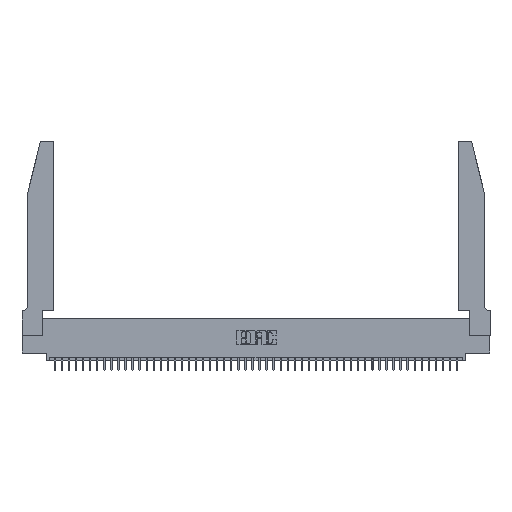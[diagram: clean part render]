
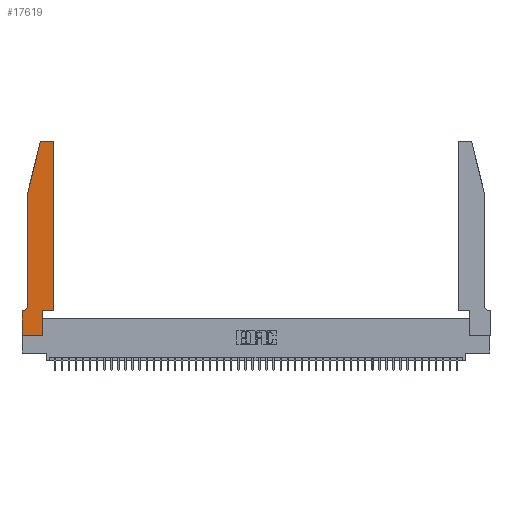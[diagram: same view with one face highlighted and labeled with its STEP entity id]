
A CAD part, top view. The second image highlights one B-rep face of the part: STEP entity #17619.
In plain terms, the highlighted planar face has unit normal (0, 0, 1).
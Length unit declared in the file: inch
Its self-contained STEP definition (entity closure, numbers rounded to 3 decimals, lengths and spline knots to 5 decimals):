
#256 = DIRECTION ( 'NONE',  ( 0., 0., 1. ) ) ;
#762 = DIRECTION ( 'NONE',  ( 0., 0., 1. ) ) ;
#788 = CARTESIAN_POINT ( 'NONE',  ( 0.4505, 0.35, 0.37 ) ) ;
#1631 = VECTOR ( 'NONE', #45136, 39.37008 ) ;
#1797 = LINE ( 'NONE', #5724, #33055 ) ;
#2536 = DIRECTION ( 'NONE',  ( 1., 0., 0. ) ) ;
#3791 = LINE ( 'NONE', #47233, #31021 ) ;
#3927 = CARTESIAN_POINT ( 'NONE',  ( 0.284, 2.72, 0.37 ) ) ;
#3953 = CARTESIAN_POINT ( 'NONE',  ( 0.4205, 2.75, 0.37 ) ) ;
#4048 = VECTOR ( 'NONE', #22663, 39.37008 ) ;
#4415 = ORIENTED_EDGE ( 'NONE', *, *, #33809, .T. ) ;
#4892 = LINE ( 'NONE', #42856, #27608 ) ;
#5573 = EDGE_CURVE ( 'NONE', #21774, #19868, #3791, .T. ) ;
#5724 = CARTESIAN_POINT ( 'NONE',  ( 0.4505, 0.35, 0.37 ) ) ;
#6302 = VERTEX_POINT ( 'NONE', #35055 ) ;
#7013 = LINE ( 'NONE', #11405, #4048 ) ;
#7291 = AXIS2_PLACEMENT_3D ( 'NONE', #7804, #34492, #30564 ) ;
#7804 = CARTESIAN_POINT ( 'NONE',  ( 0.0055, 0.42, 0.37 ) ) ;
#7945 = LINE ( 'NONE', #30465, #29139 ) ;
#7991 = EDGE_CURVE ( 'NONE', #41957, #46007, #20335, .T. ) ;
#9278 = DIRECTION ( 'NONE',  ( 1., 0., 0. ) ) ;
#9383 = CARTESIAN_POINT ( 'NONE',  ( 0.4505, 2.72, 0.37 ) ) ;
#9677 = DIRECTION ( 'NONE',  ( -1., 0., 0. ) ) ;
#10320 = EDGE_CURVE ( 'NONE', #30871, #13189, #30891, .T. ) ;
#10615 = AXIS2_PLACEMENT_3D ( 'NONE', #3927, #256, #33046 ) ;
#11405 = CARTESIAN_POINT ( 'NONE',  ( 0.0755, 2., 0.37 ) ) ;
#11772 = PLANE ( 'NONE',  #39563 ) ;
#11794 = VERTEX_POINT ( 'NONE', #34110 ) ;
#13189 = VERTEX_POINT ( 'NONE', #9383 ) ;
#13272 = VERTEX_POINT ( 'NONE', #23170 ) ;
#13441 = ORIENTED_EDGE ( 'NONE', *, *, #15421, .T. ) ;
#15421 = EDGE_CURVE ( 'NONE', #48148, #13272, #24859, .T. ) ;
#16647 = ORIENTED_EDGE ( 'NONE', *, *, #5573, .T. ) ;
#16686 = DIRECTION ( 'NONE',  ( 1., 0., 0. ) ) ;
#17405 = DIRECTION ( 'NONE',  ( -0.239, -0.971, 0. ) ) ;
#17619 = ADVANCED_FACE ( 'NONE', ( #45348 ), #11772, .T. ) ;
#19868 = VERTEX_POINT ( 'NONE', #25272 ) ;
#20249 = LINE ( 'NONE', #46697, #27808 ) ;
#20335 = LINE ( 'NONE', #39684, #27275 ) ;
#20697 = EDGE_CURVE ( 'NONE', #46007, #11794, #7013, .T. ) ;
#21774 = VERTEX_POINT ( 'NONE', #3953 ) ;
#21861 = ORIENTED_EDGE ( 'NONE', *, *, #47700, .T. ) ;
#22201 = VECTOR ( 'NONE', #9677, 39.37008 ) ;
#22219 = ORIENTED_EDGE ( 'NONE', *, *, #22561, .T. ) ;
#22561 = EDGE_CURVE ( 'NONE', #40826, #30871, #1797, .T. ) ;
#22663 = DIRECTION ( 'NONE',  ( 0., -1., 0. ) ) ;
#23170 = CARTESIAN_POINT ( 'NONE',  ( 0., 0.35, 0.37 ) ) ;
#23404 = CARTESIAN_POINT ( 'NONE',  ( 0.4505, 0.35, 0.37 ) ) ;
#24571 = VERTEX_POINT ( 'NONE', #39948 ) ;
#24859 = LINE ( 'NONE', #39808, #22201 ) ;
#25171 = DIRECTION ( 'NONE',  ( -1., 0., 0. ) ) ;
#25272 = CARTESIAN_POINT ( 'NONE',  ( 0.284, 2.75, 0.37 ) ) ;
#27260 = EDGE_CURVE ( 'NONE', #19868, #41957, #32478, .T. ) ;
#27275 = VECTOR ( 'NONE', #17405, 39.37008 ) ;
#27608 = VECTOR ( 'NONE', #9278, 39.37008 ) ;
#27808 = VECTOR ( 'NONE', #42539, 39.37008 ) ;
#28086 = DIRECTION ( 'NONE',  ( 1., 0., 0. ) ) ;
#29139 = VECTOR ( 'NONE', #45200, 39.37008 ) ;
#29678 = EDGE_LOOP ( 'NONE', ( #16647, #44611, #42166, #44431, #39946, #13441, #31675, #32362, #21861, #22219, #37811, #4415 ) ) ;
#30465 = CARTESIAN_POINT ( 'NONE',  ( 0.2865, 0.35, 0.37 ) ) ;
#30564 = DIRECTION ( 'NONE',  ( -1., 0., 0. ) ) ;
#30871 = VERTEX_POINT ( 'NONE', #23404 ) ;
#30891 = LINE ( 'NONE', #788, #1631 ) ;
#31021 = VECTOR ( 'NONE', #25171, 39.37008 ) ;
#31675 = ORIENTED_EDGE ( 'NONE', *, *, #35279, .T. ) ;
#32024 = AXIS2_PLACEMENT_3D ( 'NONE', #44183, #36590, #28086 ) ;
#32362 = ORIENTED_EDGE ( 'NONE', *, *, #44818, .T. ) ;
#32478 = CIRCLE ( 'NONE', #10615, 0.03 ) ;
#32774 = CIRCLE ( 'NONE', #32024, 0.03 ) ;
#33046 = DIRECTION ( 'NONE',  ( 1., 0., 0. ) ) ;
#33055 = VECTOR ( 'NONE', #2536, 39.37008 ) ;
#33809 = EDGE_CURVE ( 'NONE', #13189, #21774, #32774, .T. ) ;
#34110 = CARTESIAN_POINT ( 'NONE',  ( 0.0755, 0.42, 0.37 ) ) ;
#34492 = DIRECTION ( 'NONE',  ( 0., 0., -1. ) ) ;
#34617 = CARTESIAN_POINT ( 'NONE',  ( 0.2865, 0.35, 0.37 ) ) ;
#35055 = CARTESIAN_POINT ( 'NONE',  ( 0.2865, 0., 0.37 ) ) ;
#35279 = EDGE_CURVE ( 'NONE', #13272, #24571, #20249, .T. ) ;
#35457 = CIRCLE ( 'NONE', #7291, 0.07 ) ;
#36590 = DIRECTION ( 'NONE',  ( 0., 0., 1. ) ) ;
#37811 = ORIENTED_EDGE ( 'NONE', *, *, #10320, .T. ) ;
#38175 = CARTESIAN_POINT ( 'NONE',  ( 0.0055, 0.35, 0.37 ) ) ;
#39563 = AXIS2_PLACEMENT_3D ( 'NONE', #41664, #762, #16686 ) ;
#39684 = CARTESIAN_POINT ( 'NONE',  ( 0.0755, 2., 0.37 ) ) ;
#39808 = CARTESIAN_POINT ( 'NONE',  ( 0.0755, 0.35, 0.37 ) ) ;
#39946 = ORIENTED_EDGE ( 'NONE', *, *, #48145, .T. ) ;
#39948 = CARTESIAN_POINT ( 'NONE',  ( 0., 0., 0.37 ) ) ;
#40826 = VERTEX_POINT ( 'NONE', #34617 ) ;
#41664 = CARTESIAN_POINT ( 'NONE',  ( 0., 0.35, 0.37 ) ) ;
#41957 = VERTEX_POINT ( 'NONE', #47953 ) ;
#42166 = ORIENTED_EDGE ( 'NONE', *, *, #7991, .T. ) ;
#42539 = DIRECTION ( 'NONE',  ( 0., -1., 0. ) ) ;
#42856 = CARTESIAN_POINT ( 'NONE',  ( 0., 0., 0.37 ) ) ;
#44183 = CARTESIAN_POINT ( 'NONE',  ( 0.4205, 2.72, 0.37 ) ) ;
#44431 = ORIENTED_EDGE ( 'NONE', *, *, #20697, .T. ) ;
#44611 = ORIENTED_EDGE ( 'NONE', *, *, #27260, .T. ) ;
#44818 = EDGE_CURVE ( 'NONE', #24571, #6302, #4892, .T. ) ;
#45136 = DIRECTION ( 'NONE',  ( 0., 1., 0. ) ) ;
#45200 = DIRECTION ( 'NONE',  ( 0., 1., 0. ) ) ;
#45348 = FACE_OUTER_BOUND ( 'NONE', #29678, .T. ) ;
#46007 = VERTEX_POINT ( 'NONE', #47472 ) ;
#46697 = CARTESIAN_POINT ( 'NONE',  ( 0., 0., 0.37 ) ) ;
#47233 = CARTESIAN_POINT ( 'NONE',  ( 0.2605, 2.75, 0.37 ) ) ;
#47472 = CARTESIAN_POINT ( 'NONE',  ( 0.0755, 2., 0.37 ) ) ;
#47700 = EDGE_CURVE ( 'NONE', #6302, #40826, #7945, .T. ) ;
#47953 = CARTESIAN_POINT ( 'NONE',  ( 0.25487, 2.72718, 0.37 ) ) ;
#48145 = EDGE_CURVE ( 'NONE', #11794, #48148, #35457, .T. ) ;
#48148 = VERTEX_POINT ( 'NONE', #38175 ) ;
